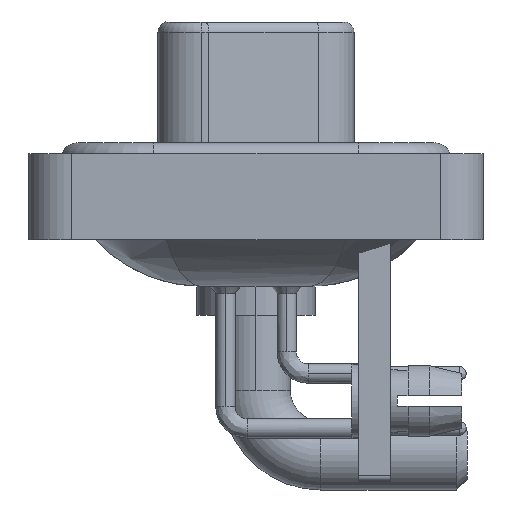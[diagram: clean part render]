
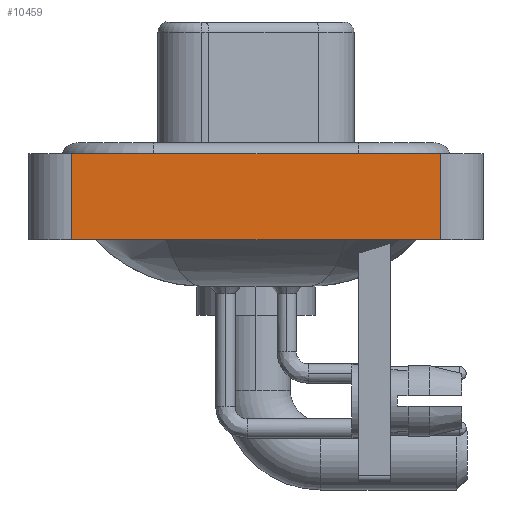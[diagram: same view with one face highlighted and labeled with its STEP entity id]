
A CAD part, left-side view. The second image highlights one B-rep face of the part: STEP entity #10459.
In plain terms, the highlighted planar face has unit normal (-1, 0, 0).
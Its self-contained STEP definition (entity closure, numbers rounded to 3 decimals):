
#678 = VERTEX_POINT ( 'NONE', #785 ) ;
#785 = CARTESIAN_POINT ( 'NONE',  ( -7.3, -8.55, 0.4 ) ) ;
#1317 = VECTOR ( 'NONE', #16650, 1000. ) ;
#2172 = CARTESIAN_POINT ( 'NONE',  ( -7.3, -8.55, -3.6 ) ) ;
#2277 = DIRECTION ( 'NONE',  ( 0., -1., 0. ) ) ;
#3909 = PLANE ( 'NONE',  #16380 ) ;
#4331 = FACE_OUTER_BOUND ( 'NONE', #8418, .T. ) ;
#4434 = CARTESIAN_POINT ( 'NONE',  ( -7.3, -8.55, 0.4 ) ) ;
#4577 = EDGE_CURVE ( 'NONE', #24001, #678, #7161, .T. ) ;
#4639 = CARTESIAN_POINT ( 'NONE',  ( -7.3, -8.55, -3.6 ) ) ;
#4733 = ORIENTED_EDGE ( 'NONE', *, *, #4577, .F. ) ;
#4939 = CARTESIAN_POINT ( 'NONE',  ( -7.3, 8.55, -3.6 ) ) ;
#5635 = VECTOR ( 'NONE', #2277, 1000. ) ;
#6104 = CARTESIAN_POINT ( 'NONE',  ( -7.3, 8.55, 0.4 ) ) ;
#7161 = LINE ( 'NONE', #4434, #5635 ) ;
#8418 = EDGE_LOOP ( 'NONE', ( #15642, #4733, #14042, #26188 ) ) ;
#10112 = VERTEX_POINT ( 'NONE', #4639 ) ;
#10193 = LINE ( 'NONE', #18937, #23748 ) ;
#10459 = ADVANCED_FACE ( 'NONE', ( #4331 ), #3909, .T. ) ;
#10799 = DIRECTION ( 'NONE',  ( -1., 0., 0. ) ) ;
#11368 = CARTESIAN_POINT ( 'NONE',  ( -7.3, -8.55, -3.6 ) ) ;
#14042 = ORIENTED_EDGE ( 'NONE', *, *, #25730, .F. ) ;
#15642 = ORIENTED_EDGE ( 'NONE', *, *, #25696, .T. ) ;
#15658 = LINE ( 'NONE', #11368, #21465 ) ;
#16380 = AXIS2_PLACEMENT_3D ( 'NONE', #2172, #10799, #28150 ) ;
#16650 = DIRECTION ( 'NONE',  ( 0., 0., 1. ) ) ;
#18937 = CARTESIAN_POINT ( 'NONE',  ( -7.3, -8.55, -3.6 ) ) ;
#19237 = DIRECTION ( 'NONE',  ( 0., 0., 1. ) ) ;
#20113 = DIRECTION ( 'NONE',  ( 0., -1., 0. ) ) ;
#20874 = VERTEX_POINT ( 'NONE', #4939 ) ;
#20963 = LINE ( 'NONE', #21377, #1317 ) ;
#21377 = CARTESIAN_POINT ( 'NONE',  ( -7.3, 8.55, -3.6 ) ) ;
#21465 = VECTOR ( 'NONE', #20113, 1000. ) ;
#23748 = VECTOR ( 'NONE', #19237, 1000. ) ;
#24001 = VERTEX_POINT ( 'NONE', #6104 ) ;
#25554 = EDGE_CURVE ( 'NONE', #20874, #10112, #15658, .T. ) ;
#25696 = EDGE_CURVE ( 'NONE', #10112, #678, #10193, .T. ) ;
#25730 = EDGE_CURVE ( 'NONE', #20874, #24001, #20963, .T. ) ;
#26188 = ORIENTED_EDGE ( 'NONE', *, *, #25554, .T. ) ;
#28150 = DIRECTION ( 'NONE',  ( 0., 0., 1. ) ) ;
